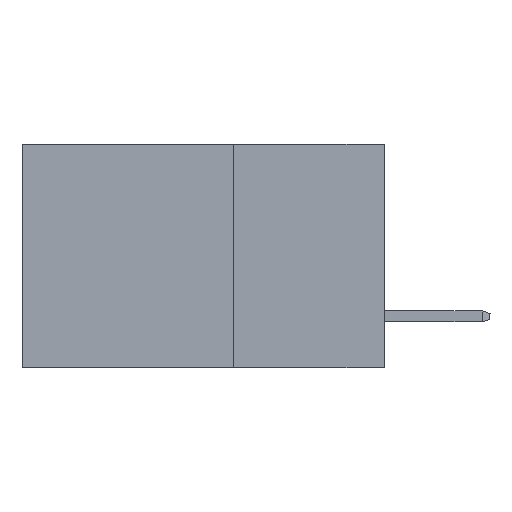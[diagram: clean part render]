
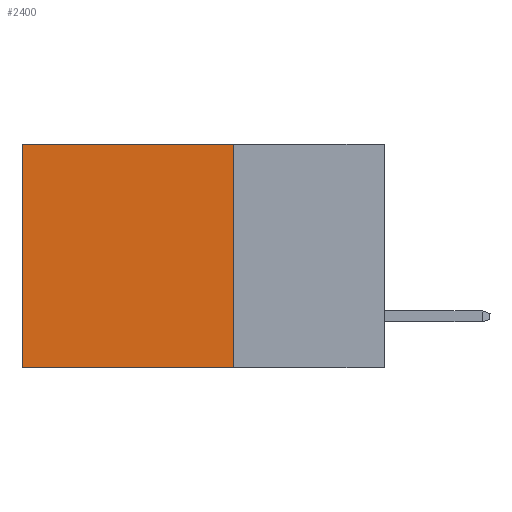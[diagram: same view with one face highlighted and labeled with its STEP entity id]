
A CAD part, left-side view. The second image highlights one B-rep face of the part: STEP entity #2400.
In plain terms, the highlighted planar face has unit normal (-1, 0, 0).
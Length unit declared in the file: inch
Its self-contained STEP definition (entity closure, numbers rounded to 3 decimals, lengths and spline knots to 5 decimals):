
#420 = EDGE_CURVE ( 'NONE', #21701, #13662, #4868, .T. ) ;
#1256 = VERTEX_POINT ( 'NONE', #20579 ) ;
#2130 = CARTESIAN_POINT ( 'NONE',  ( 0.2615, 0.6, 0. ) ) ;
#2400 = ADVANCED_FACE ( 'NONE', ( #9869 ), #12051, .F. ) ;
#2734 = CARTESIAN_POINT ( 'NONE',  ( 0.2615, 0.25, -0.37 ) ) ;
#2766 = DIRECTION ( 'NONE',  ( 0., 1., 0. ) ) ;
#2884 = CARTESIAN_POINT ( 'NONE',  ( 0.2615, 0.25, -0.37 ) ) ;
#4253 = EDGE_CURVE ( 'NONE', #6118, #13662, #16482, .T. ) ;
#4868 = LINE ( 'NONE', #20513, #16799 ) ;
#5338 = EDGE_CURVE ( 'NONE', #1256, #21701, #9505, .T. ) ;
#6118 = VERTEX_POINT ( 'NONE', #21056 ) ;
#6342 = EDGE_LOOP ( 'NONE', ( #19111, #10248, #20690, #6661 ) ) ;
#6460 = VECTOR ( 'NONE', #2766, 39.37008 ) ;
#6661 = ORIENTED_EDGE ( 'NONE', *, *, #5338, .T. ) ;
#7336 = DIRECTION ( 'NONE',  ( 0., 0., -1. ) ) ;
#8685 = CARTESIAN_POINT ( 'NONE',  ( 0.2615, 0.25, -0.37 ) ) ;
#9007 = EDGE_CURVE ( 'NONE', #1256, #6118, #21959, .T. ) ;
#9505 = LINE ( 'NONE', #17314, #21504 ) ;
#9869 = FACE_OUTER_BOUND ( 'NONE', #6342, .T. ) ;
#10237 = DIRECTION ( 'NONE',  ( 1., 0., 0. ) ) ;
#10248 = ORIENTED_EDGE ( 'NONE', *, *, #4253, .F. ) ;
#12051 = PLANE ( 'NONE',  #25247 ) ;
#13662 = VERTEX_POINT ( 'NONE', #16550 ) ;
#14959 = VECTOR ( 'NONE', #16334, 39.37008 ) ;
#16334 = DIRECTION ( 'NONE',  ( 0., 0., -1. ) ) ;
#16482 = LINE ( 'NONE', #2884, #6460 ) ;
#16550 = CARTESIAN_POINT ( 'NONE',  ( 0.2615, 0.6, -0.37 ) ) ;
#16799 = VECTOR ( 'NONE', #7336, 39.37008 ) ;
#17314 = CARTESIAN_POINT ( 'NONE',  ( 0.2615, 0.25, 0. ) ) ;
#19111 = ORIENTED_EDGE ( 'NONE', *, *, #420, .T. ) ;
#20513 = CARTESIAN_POINT ( 'NONE',  ( 0.2615, 0.6, -0.37 ) ) ;
#20579 = CARTESIAN_POINT ( 'NONE',  ( 0.2615, 0.25, 0. ) ) ;
#20690 = ORIENTED_EDGE ( 'NONE', *, *, #9007, .F. ) ;
#21056 = CARTESIAN_POINT ( 'NONE',  ( 0.2615, 0.25, -0.37 ) ) ;
#21504 = VECTOR ( 'NONE', #25066, 39.37008 ) ;
#21701 = VERTEX_POINT ( 'NONE', #2130 ) ;
#21959 = LINE ( 'NONE', #2734, #14959 ) ;
#23770 = DIRECTION ( 'NONE',  ( 0., 0., -1. ) ) ;
#25066 = DIRECTION ( 'NONE',  ( 0., 1., 0. ) ) ;
#25247 = AXIS2_PLACEMENT_3D ( 'NONE', #8685, #10237, #23770 ) ;
